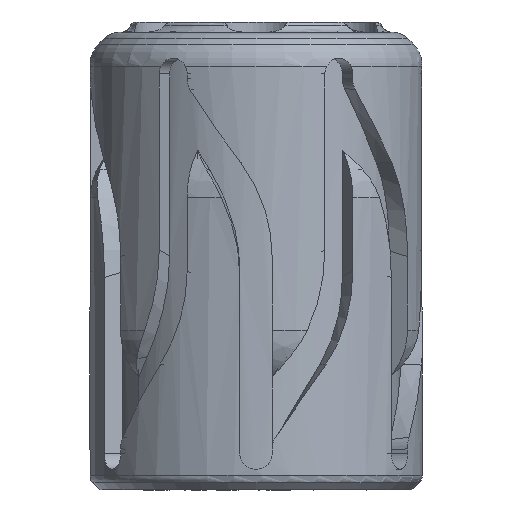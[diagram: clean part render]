
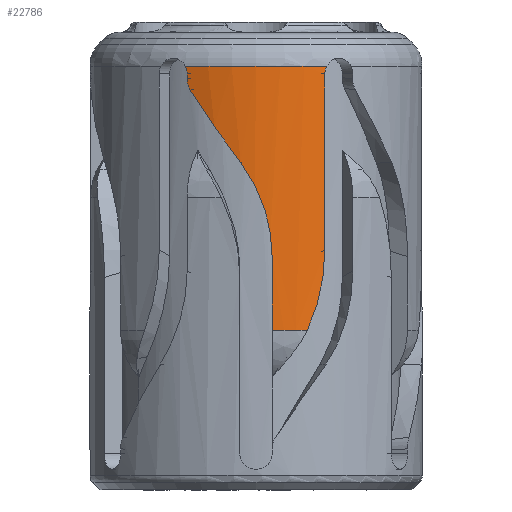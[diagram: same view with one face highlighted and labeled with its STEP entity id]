
A CAD part, front view. The second image highlights one B-rep face of the part: STEP entity #22786.
In plain terms, the highlighted cylindrical face has radius 16 mm (diameter 32 mm), a partial arc.
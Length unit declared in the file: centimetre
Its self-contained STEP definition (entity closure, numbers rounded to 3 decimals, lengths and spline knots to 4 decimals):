
#1176=LINE($,#34149,#1680);
#1177=LINE($,#34175,#1681);
#1178=LINE($,#34193,#1682);
#1680=VECTOR($,#26259,0.0453);
#1681=VECTOR($,#26260,0.7075);
#1682=VECTOR($,#26263,1.6937);
#2092=CYLINDRICAL_SURFACE($,#24192,1.6);
#2845=B_SPLINE_CURVE_WITH_KNOTS($,3,(#34142,#34143,#34144,#34145,#34146,
#34147),.UNSPECIFIED.,.F.,.F.,(4,2,4),(0.3766,0.3958,
0.4523),.UNSPECIFIED.);
#2846=B_SPLINE_CURVE_WITH_KNOTS($,3,(#34151,#34152,#34153,#34154,#34155,
#34156,#34157),.UNSPECIFIED.,.F.,.F.,(4,3,4),(0.,0.0586,0.1171),
 .UNSPECIFIED.);
#2847=B_SPLINE_CURVE_WITH_KNOTS($,3,(#34159,#34160,#34161,#34162,#34163,
#34164),.UNSPECIFIED.,.F.,.F.,(4,2,4),(0.0292,0.3893,
0.8895),.UNSPECIFIED.);
#2848=B_SPLINE_CURVE_WITH_KNOTS($,3,(#34166,#34167,#34168,#34169,#34170,
#34171,#34172,#34173),.UNSPECIFIED.,.F.,.F.,(4,2,2,4),(0.,0.3732,
0.6655,0.9725),.UNSPECIFIED.);
#2849=B_SPLINE_CURVE_WITH_KNOTS($,3,(#34179,#34180,#34181,#34182,#34183,
#34184,#34185,#34186,#34187,#34188,#34189,#34190,#34191),.UNSPECIFIED.,
 .F.,.F.,(4,3,3,3,4),(0.3306,0.3653,0.607,
0.7289,1.1292),.UNSPECIFIED.);
#2850=B_SPLINE_CURVE_WITH_KNOTS($,3,(#34194,#34195,#34196,#34197,#34198,
#34199),.UNSPECIFIED.,.F.,.F.,(4,2,4),(0.4523,0.5089,
0.5281),.UNSPECIFIED.);
#5109=FACE_OUTER_BOUND($,#6479,.T.);
#6479=EDGE_LOOP($,(#16091,#16092,#16093,#16094,#16095,#16096,#16097,#16098,
#16099,#16100,#16101));
#7826=CIRCLE($,#24174,1.6);
#7833=CIRCLE($,#24193,1.6);
#8956=VERTEX_POINT($,#33874);
#8957=VERTEX_POINT($,#33887);
#8992=VERTEX_POINT($,#34141);
#8993=VERTEX_POINT($,#34148);
#8994=VERTEX_POINT($,#34150);
#8995=VERTEX_POINT($,#34158);
#8996=VERTEX_POINT($,#34165);
#8997=VERTEX_POINT($,#34174);
#8998=VERTEX_POINT($,#34176);
#8999=VERTEX_POINT($,#34178);
#9000=VERTEX_POINT($,#34192);
#11656=EDGE_CURVE($,#8956,#8957,#7826,.T.);
#11703=EDGE_CURVE($,#8956,#8992,#2845,.T.);
#11704=EDGE_CURVE($,#8992,#8993,#1176,.T.);
#11705=EDGE_CURVE($,#8993,#8994,#2846,.T.);
#11706=EDGE_CURVE($,#8994,#8995,#2847,.T.);
#11707=EDGE_CURVE($,#8995,#8996,#2848,.T.);
#11708=EDGE_CURVE($,#8996,#8997,#1177,.T.);
#11709=EDGE_CURVE($,#8998,#8997,#7833,.T.);
#11710=EDGE_CURVE($,#8998,#8999,#2849,.T.);
#11711=EDGE_CURVE($,#8999,#9000,#1178,.T.);
#11712=EDGE_CURVE($,#9000,#8957,#2850,.T.);
#16091=ORIENTED_EDGE($,*,*,#11656,.F.);
#16092=ORIENTED_EDGE($,*,*,#11703,.T.);
#16093=ORIENTED_EDGE($,*,*,#11704,.T.);
#16094=ORIENTED_EDGE($,*,*,#11705,.T.);
#16095=ORIENTED_EDGE($,*,*,#11706,.T.);
#16096=ORIENTED_EDGE($,*,*,#11707,.T.);
#16097=ORIENTED_EDGE($,*,*,#11708,.T.);
#16098=ORIENTED_EDGE($,*,*,#11709,.F.);
#16099=ORIENTED_EDGE($,*,*,#11710,.T.);
#16100=ORIENTED_EDGE($,*,*,#11711,.T.);
#16101=ORIENTED_EDGE($,*,*,#11712,.T.);
#22786=ADVANCED_FACE($,(#5109),#2092,.T.);
#24174=AXIS2_PLACEMENT_3D($,#33888,#26203,#26204);
#24192=AXIS2_PLACEMENT_3D($,#34140,#26257,#26258);
#24193=AXIS2_PLACEMENT_3D($,#34177,#26261,#26262);
#26203=DIRECTION('center_axis',(0.,0.,1.));
#26204=DIRECTION('ref_axis',(-1.,0.,0.));
#26257=DIRECTION('center_axis',(0.,0.,-1.));
#26258=DIRECTION('ref_axis',(-1.,0.,0.));
#26259=DIRECTION($,(0.,0.,-1.));
#26260=DIRECTION($,(0.,0.,-1.));
#26261=DIRECTION('center_axis',(0.,0.,-1.));
#26262=DIRECTION('ref_axis',(0.158,-0.987,0.));
#26263=DIRECTION($,(0.,0.,1.));
#33874=CARTESIAN_POINT('',(-4.1257,1.6304,4.2907));
#33887=CARTESIAN_POINT('',(-2.7643,1.6304,4.2907));
#33888=CARTESIAN_POINT('Origin',(-3.445,3.0785,4.2907));
#34140=CARTESIAN_POINT('Origin',(-3.445,3.0785,0.465));
#34141=CARTESIAN_POINT('',(-4.107,1.6218,4.2151));
#34142=CARTESIAN_POINT('Ctrl Pts',(-4.1257,1.6304,4.2907));
#34143=CARTESIAN_POINT('Ctrl Pts',(-4.1226,1.629,4.2849));
#34144=CARTESIAN_POINT('Ctrl Pts',(-4.1198,1.6277,4.2788));
#34145=CARTESIAN_POINT('Ctrl Pts',(-4.1105,1.6234,4.254));
#34146=CARTESIAN_POINT('Ctrl Pts',(-4.107,1.6218,4.234));
#34147=CARTESIAN_POINT('Ctrl Pts',(-4.107,1.6218,4.2151));
#34148=CARTESIAN_POINT('',(-4.107,1.6218,4.1698));
#34149=CARTESIAN_POINT($,(-4.107,1.6218,0.465));
#34150=CARTESIAN_POINT('',(-4.0765,1.6083,4.0595));
#34151=CARTESIAN_POINT('Ctrl Pts',(-4.107,1.6218,4.1698));
#34152=CARTESIAN_POINT('Ctrl Pts',(-4.107,1.6218,4.1503));
#34153=CARTESIAN_POINT('Ctrl Pts',(-4.1043,1.6206,4.1309));
#34154=CARTESIAN_POINT('Ctrl Pts',(-4.0992,1.6183,4.1122));
#34155=CARTESIAN_POINT('Ctrl Pts',(-4.094,1.616,4.0935));
#34156=CARTESIAN_POINT('Ctrl Pts',(-4.0864,1.6126,4.0757));
#34157=CARTESIAN_POINT('Ctrl Pts',(-4.0765,1.6083,4.0595));
#34158=CARTESIAN_POINT('',(-3.5938,1.4854,3.3638));
#34159=CARTESIAN_POINT('Ctrl Pts',(-4.0765,1.6083,4.0595));
#34160=CARTESIAN_POINT('Ctrl Pts',(-4.0153,1.5821,3.9598));
#34161=CARTESIAN_POINT('Ctrl Pts',(-3.951,1.5589,3.8621));
#34162=CARTESIAN_POINT('Ctrl Pts',(-3.7902,1.5131,3.6292));
#34163=CARTESIAN_POINT('Ctrl Pts',(-3.6932,1.4947,3.4973));
#34164=CARTESIAN_POINT('Ctrl Pts',(-3.5938,1.4854,3.3638));
#34165=CARTESIAN_POINT('',(-3.29,1.486,2.459));
#34166=CARTESIAN_POINT('Ctrl Pts',(-3.5938,1.4854,3.3638));
#34167=CARTESIAN_POINT('Ctrl Pts',(-3.5197,1.4785,3.2641));
#34168=CARTESIAN_POINT('Ctrl Pts',(-3.4573,1.4778,3.1566));
#34169=CARTESIAN_POINT('Ctrl Pts',(-3.3706,1.4797,2.9522));
#34170=CARTESIAN_POINT('Ctrl Pts',(-3.3413,1.4817,2.8591));
#34171=CARTESIAN_POINT('Ctrl Pts',(-3.3005,1.4849,2.6634));
#34172=CARTESIAN_POINT('Ctrl Pts',(-3.29,1.486,2.5614));
#34173=CARTESIAN_POINT('Ctrl Pts',(-3.29,1.486,2.459));
#34174=CARTESIAN_POINT('',(-3.29,1.486,1.7515));
#34175=CARTESIAN_POINT($,(-3.29,1.486,0.465));
#34176=CARTESIAN_POINT('',(-2.9522,1.5562,1.7515));
#34177=CARTESIAN_POINT('Origin',(-3.445,3.0785,1.7515));
#34178=CARTESIAN_POINT('',(-2.783,1.6218,2.5214));
#34179=CARTESIAN_POINT('Ctrl Pts',(-2.9522,1.5561,1.7515));
#34180=CARTESIAN_POINT('Ctrl Pts',(-2.9474,1.5577,1.7618));
#34181=CARTESIAN_POINT('Ctrl Pts',(-2.9426,1.5593,1.7723));
#34182=CARTESIAN_POINT('Ctrl Pts',(-2.9379,1.5608,1.7827));
#34183=CARTESIAN_POINT('Ctrl Pts',(-2.9054,1.5717,1.8556));
#34184=CARTESIAN_POINT('Ctrl Pts',(-2.8779,1.5821,1.9307));
#34185=CARTESIAN_POINT('Ctrl Pts',(-2.8555,1.5909,2.0074));
#34186=CARTESIAN_POINT('Ctrl Pts',(-2.8443,1.5954,2.0461));
#34187=CARTESIAN_POINT('Ctrl Pts',(-2.8343,1.5995,2.0853));
#34188=CARTESIAN_POINT('Ctrl Pts',(-2.8257,1.6032,2.1249));
#34189=CARTESIAN_POINT('Ctrl Pts',(-2.7973,1.6151,2.2548));
#34190=CARTESIAN_POINT('Ctrl Pts',(-2.783,1.6218,2.3879));
#34191=CARTESIAN_POINT('Ctrl Pts',(-2.783,1.6218,2.5214));
#34192=CARTESIAN_POINT('',(-2.783,1.6218,4.2151));
#34193=CARTESIAN_POINT($,(-2.783,1.6218,0.465));
#34194=CARTESIAN_POINT('Ctrl Pts',(-2.783,1.6218,4.2151));
#34195=CARTESIAN_POINT('Ctrl Pts',(-2.783,1.6218,4.234));
#34196=CARTESIAN_POINT('Ctrl Pts',(-2.7795,1.6234,4.254));
#34197=CARTESIAN_POINT('Ctrl Pts',(-2.7702,1.6277,4.2788));
#34198=CARTESIAN_POINT('Ctrl Pts',(-2.7674,1.629,4.2849));
#34199=CARTESIAN_POINT('Ctrl Pts',(-2.7643,1.6304,4.2907));
